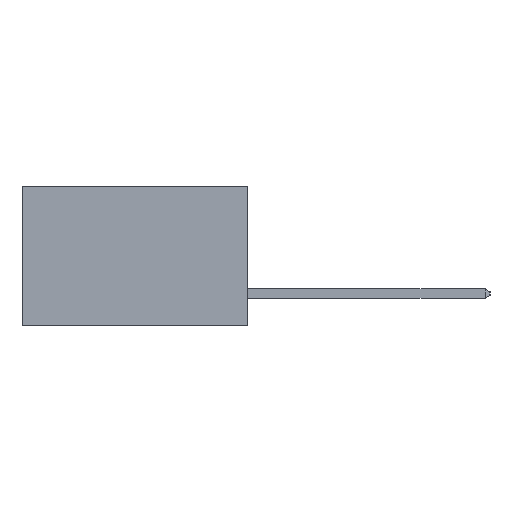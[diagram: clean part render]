
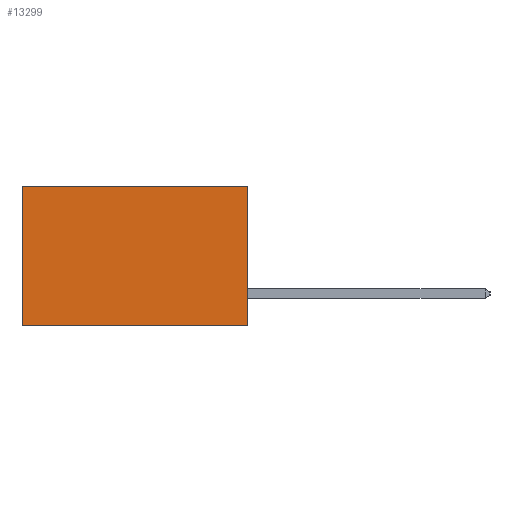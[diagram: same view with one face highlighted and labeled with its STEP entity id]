
A CAD part, left-side view. The second image highlights one B-rep face of the part: STEP entity #13299.
In plain terms, the highlighted planar face has unit normal (-1, 0, 0).
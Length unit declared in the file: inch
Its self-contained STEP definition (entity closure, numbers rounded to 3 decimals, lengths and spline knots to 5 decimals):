
#680 = ORIENTED_EDGE ( 'NONE', *, *, #19610, .F. ) ;
#1254 = VERTEX_POINT ( 'NONE', #5486 ) ;
#1391 = AXIS2_PLACEMENT_3D ( 'NONE', #18631, #20468, #9472 ) ;
#2605 = VECTOR ( 'NONE', #12277, 39.37008 ) ;
#3471 = DIRECTION ( 'NONE',  ( 0., 1., 0. ) ) ;
#3842 = DIRECTION ( 'NONE',  ( 0., 0., -1. ) ) ;
#4334 = LINE ( 'NONE', #24141, #23452 ) ;
#4514 = VERTEX_POINT ( 'NONE', #9061 ) ;
#5486 = CARTESIAN_POINT ( 'NONE',  ( 0.298, 0.6, 0. ) ) ;
#5632 = PLANE ( 'NONE',  #1391 ) ;
#5765 = DIRECTION ( 'NONE',  ( 0., 0., -1. ) ) ;
#9061 = CARTESIAN_POINT ( 'NONE',  ( 0.298, 0., 0. ) ) ;
#9472 = DIRECTION ( 'NONE',  ( 0., 0., -1. ) ) ;
#9581 = VERTEX_POINT ( 'NONE', #23610 ) ;
#10361 = CARTESIAN_POINT ( 'NONE',  ( 0.298, 0., -0.37 ) ) ;
#10680 = ORIENTED_EDGE ( 'NONE', *, *, #13219, .T. ) ;
#12181 = VERTEX_POINT ( 'NONE', #17354 ) ;
#12277 = DIRECTION ( 'NONE',  ( 0., 1., 0. ) ) ;
#12319 = EDGE_CURVE ( 'NONE', #12181, #9581, #13325, .T. ) ;
#12358 = ORIENTED_EDGE ( 'NONE', *, *, #12319, .F. ) ;
#12639 = ORIENTED_EDGE ( 'NONE', *, *, #21587, .T. ) ;
#13219 = EDGE_CURVE ( 'NONE', #4514, #1254, #15171, .T. ) ;
#13299 = ADVANCED_FACE ( 'NONE', ( #22003 ), #5632, .F. ) ;
#13306 = CARTESIAN_POINT ( 'NONE',  ( 0.298, 0., 0. ) ) ;
#13325 = LINE ( 'NONE', #10361, #2605 ) ;
#14499 = EDGE_LOOP ( 'NONE', ( #12639, #12358, #680, #10680 ) ) ;
#15171 = LINE ( 'NONE', #22094, #19040 ) ;
#16477 = VECTOR ( 'NONE', #5765, 39.37008 ) ;
#17027 = LINE ( 'NONE', #13306, #16477 ) ;
#17354 = CARTESIAN_POINT ( 'NONE',  ( 0.298, 0., -0.37 ) ) ;
#18631 = CARTESIAN_POINT ( 'NONE',  ( 0.298, 0., 0. ) ) ;
#19040 = VECTOR ( 'NONE', #3471, 39.37008 ) ;
#19610 = EDGE_CURVE ( 'NONE', #4514, #12181, #17027, .T. ) ;
#20468 = DIRECTION ( 'NONE',  ( 1., 0., 0. ) ) ;
#21587 = EDGE_CURVE ( 'NONE', #1254, #9581, #4334, .T. ) ;
#22003 = FACE_OUTER_BOUND ( 'NONE', #14499, .T. ) ;
#22094 = CARTESIAN_POINT ( 'NONE',  ( 0.298, 0., 0. ) ) ;
#23452 = VECTOR ( 'NONE', #3842, 39.37008 ) ;
#23610 = CARTESIAN_POINT ( 'NONE',  ( 0.298, 0.6, -0.37 ) ) ;
#24141 = CARTESIAN_POINT ( 'NONE',  ( 0.298, 0.6, 0. ) ) ;
